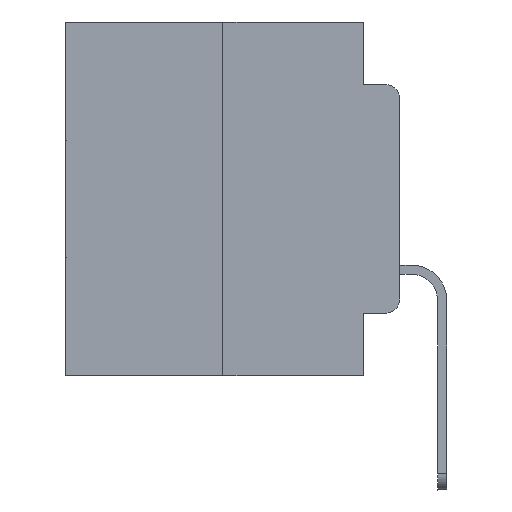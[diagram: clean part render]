
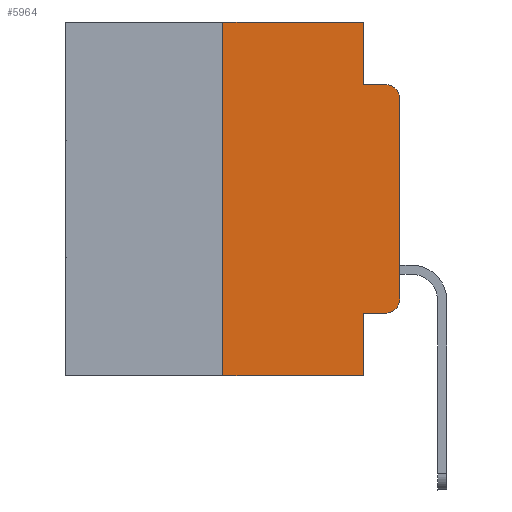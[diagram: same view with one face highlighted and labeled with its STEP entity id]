
A CAD part, left-side view. The second image highlights one B-rep face of the part: STEP entity #5964.
In plain terms, the highlighted planar face has unit normal (-1, 0, 0).
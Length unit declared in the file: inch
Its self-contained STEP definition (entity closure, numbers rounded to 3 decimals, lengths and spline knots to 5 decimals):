
#157 = CARTESIAN_POINT ( 'NONE',  ( 0., 0.02, -0.0885 ) ) ;
#253 = CARTESIAN_POINT ( 'NONE',  ( 0., 0.02, -0.3915 ) ) ;
#2045 = EDGE_CURVE ( 'NONE', #20629, #19738, #24509, .T. ) ;
#2225 = DIRECTION ( 'NONE',  ( 0., 0., -1. ) ) ;
#2373 = FACE_OUTER_BOUND ( 'NONE', #26656, .T. ) ;
#2468 = DIRECTION ( 'NONE',  ( 0., 0., -1. ) ) ;
#2503 = DIRECTION ( 'NONE',  ( 0., 0., -1. ) ) ;
#2640 = VERTEX_POINT ( 'NONE', #24760 ) ;
#2712 = AXIS2_PLACEMENT_3D ( 'NONE', #21575, #6403, #2468 ) ;
#2785 = VERTEX_POINT ( 'NONE', #25860 ) ;
#3186 = DIRECTION ( 'NONE',  ( 0., -1., 0. ) ) ;
#3329 = VECTOR ( 'NONE', #17908, 39.37008 ) ;
#3701 = EDGE_CURVE ( 'NONE', #19738, #9041, #19016, .T. ) ;
#3760 = CARTESIAN_POINT ( 'NONE',  ( 0., 0., 0. ) ) ;
#4982 = ORIENTED_EDGE ( 'NONE', *, *, #11864, .T. ) ;
#5471 = CARTESIAN_POINT ( 'NONE',  ( 0., 0.25, -0.5 ) ) ;
#5964 = ADVANCED_FACE ( 'NONE', ( #2373 ), #6579, .F. ) ;
#6244 = VERTEX_POINT ( 'NONE', #14404 ) ;
#6335 = DIRECTION ( 'NONE',  ( 0., -1., 0. ) ) ;
#6403 = DIRECTION ( 'NONE',  ( -1., 0., 0. ) ) ;
#6542 = ORIENTED_EDGE ( 'NONE', *, *, #26681, .T. ) ;
#6579 = PLANE ( 'NONE',  #8181 ) ;
#7123 = CIRCLE ( 'NONE', #21925, 0.02 ) ;
#7400 = CARTESIAN_POINT ( 'NONE',  ( 0., 0.473, -0.5 ) ) ;
#7639 = VERTEX_POINT ( 'NONE', #24452 ) ;
#8181 = AXIS2_PLACEMENT_3D ( 'NONE', #19513, #17661, #2503 ) ;
#8368 = LINE ( 'NONE', #3760, #10587 ) ;
#8714 = CARTESIAN_POINT ( 'NONE',  ( 0., 0.051, -0.4115 ) ) ;
#9041 = VERTEX_POINT ( 'NONE', #12492 ) ;
#9210 = CARTESIAN_POINT ( 'NONE',  ( 0., 0.25, 0. ) ) ;
#9380 = ORIENTED_EDGE ( 'NONE', *, *, #25182, .F. ) ;
#9641 = LINE ( 'NONE', #7400, #21034 ) ;
#9655 = EDGE_CURVE ( 'NONE', #6244, #25053, #12869, .T. ) ;
#9778 = LINE ( 'NONE', #18353, #24606 ) ;
#10587 = VECTOR ( 'NONE', #14399, 39.37008 ) ;
#11069 = EDGE_CURVE ( 'NONE', #7639, #2640, #8368, .T. ) ;
#11159 = EDGE_CURVE ( 'NONE', #9041, #2785, #26220, .T. ) ;
#11177 = DIRECTION ( 'NONE',  ( -1., 0., 0. ) ) ;
#11797 = ORIENTED_EDGE ( 'NONE', *, *, #2045, .F. ) ;
#11864 = EDGE_CURVE ( 'NONE', #6244, #26542, #23752, .T. ) ;
#12314 = ORIENTED_EDGE ( 'NONE', *, *, #9655, .F. ) ;
#12386 = DIRECTION ( 'NONE',  ( 0., -1., 0. ) ) ;
#12492 = CARTESIAN_POINT ( 'NONE',  ( 0., 0.051, 0. ) ) ;
#12869 = LINE ( 'NONE', #21469, #19515 ) ;
#12995 = CIRCLE ( 'NONE', #2712, 0.02 ) ;
#13270 = DIRECTION ( 'NONE',  ( 0., 0., -1. ) ) ;
#13296 = VECTOR ( 'NONE', #6335, 39.37008 ) ;
#13836 = CARTESIAN_POINT ( 'NONE',  ( 0., 0.25, 0. ) ) ;
#14399 = DIRECTION ( 'NONE',  ( 0., 0., 1. ) ) ;
#14404 = CARTESIAN_POINT ( 'NONE',  ( 0., 0.051, -0.4115 ) ) ;
#15246 = VECTOR ( 'NONE', #12386, 39.37008 ) ;
#17227 = CARTESIAN_POINT ( 'NONE',  ( 0., 0.051, -0.5 ) ) ;
#17508 = DIRECTION ( 'NONE',  ( 0., 0., -1. ) ) ;
#17661 = DIRECTION ( 'NONE',  ( 1., 0., 0. ) ) ;
#17901 = ORIENTED_EDGE ( 'NONE', *, *, #25118, .T. ) ;
#17908 = DIRECTION ( 'NONE',  ( 0., 0., 1. ) ) ;
#18353 = CARTESIAN_POINT ( 'NONE',  ( 0., 0.051, -0.0885 ) ) ;
#19016 = LINE ( 'NONE', #25740, #15246 ) ;
#19216 = ORIENTED_EDGE ( 'NONE', *, *, #3701, .F. ) ;
#19513 = CARTESIAN_POINT ( 'NONE',  ( 0., 0.473, 0. ) ) ;
#19515 = VECTOR ( 'NONE', #2225, 39.37008 ) ;
#19738 = VERTEX_POINT ( 'NONE', #13836 ) ;
#20027 = VECTOR ( 'NONE', #17508, 39.37008 ) ;
#20629 = VERTEX_POINT ( 'NONE', #5471 ) ;
#21034 = VECTOR ( 'NONE', #22280, 39.37008 ) ;
#21209 = ORIENTED_EDGE ( 'NONE', *, *, #11159, .F. ) ;
#21469 = CARTESIAN_POINT ( 'NONE',  ( 0., 0.051, 0. ) ) ;
#21575 = CARTESIAN_POINT ( 'NONE',  ( 0., 0.02, -0.1085 ) ) ;
#21692 = ORIENTED_EDGE ( 'NONE', *, *, #23670, .T. ) ;
#21925 = AXIS2_PLACEMENT_3D ( 'NONE', #253, #11177, #13270 ) ;
#22280 = DIRECTION ( 'NONE',  ( 0., -1., 0. ) ) ;
#22596 = ORIENTED_EDGE ( 'NONE', *, *, #11069, .T. ) ;
#23670 = EDGE_CURVE ( 'NONE', #26542, #7639, #7123, .T. ) ;
#23752 = LINE ( 'NONE', #8714, #13296 ) ;
#24452 = CARTESIAN_POINT ( 'NONE',  ( 0., 0., -0.3915 ) ) ;
#24509 = LINE ( 'NONE', #9210, #3329 ) ;
#24594 = VERTEX_POINT ( 'NONE', #157 ) ;
#24606 = VECTOR ( 'NONE', #3186, 39.37008 ) ;
#24760 = CARTESIAN_POINT ( 'NONE',  ( 0., 0., -0.1085 ) ) ;
#25053 = VERTEX_POINT ( 'NONE', #17227 ) ;
#25118 = EDGE_CURVE ( 'NONE', #20629, #25053, #9641, .T. ) ;
#25182 = EDGE_CURVE ( 'NONE', #2785, #24594, #9778, .T. ) ;
#25740 = CARTESIAN_POINT ( 'NONE',  ( 0., 0.473, 0. ) ) ;
#25860 = CARTESIAN_POINT ( 'NONE',  ( 0., 0.051, -0.0885 ) ) ;
#26220 = LINE ( 'NONE', #26355, #20027 ) ;
#26355 = CARTESIAN_POINT ( 'NONE',  ( 0., 0.051, 0. ) ) ;
#26542 = VERTEX_POINT ( 'NONE', #27622 ) ;
#26656 = EDGE_LOOP ( 'NONE', ( #22596, #6542, #9380, #21209, #19216, #11797, #17901, #12314, #4982, #21692 ) ) ;
#26681 = EDGE_CURVE ( 'NONE', #2640, #24594, #12995, .T. ) ;
#27622 = CARTESIAN_POINT ( 'NONE',  ( 0., 0.02, -0.4115 ) ) ;
